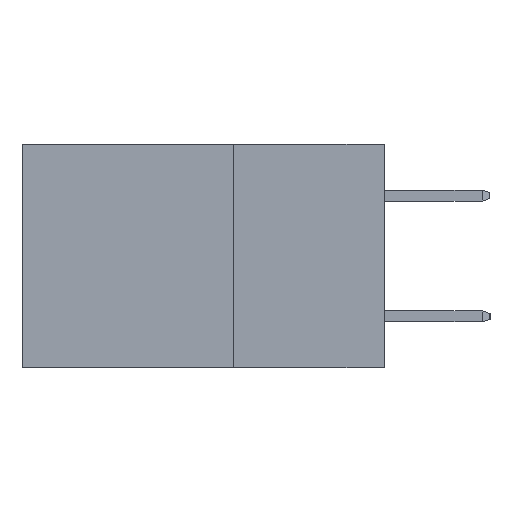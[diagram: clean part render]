
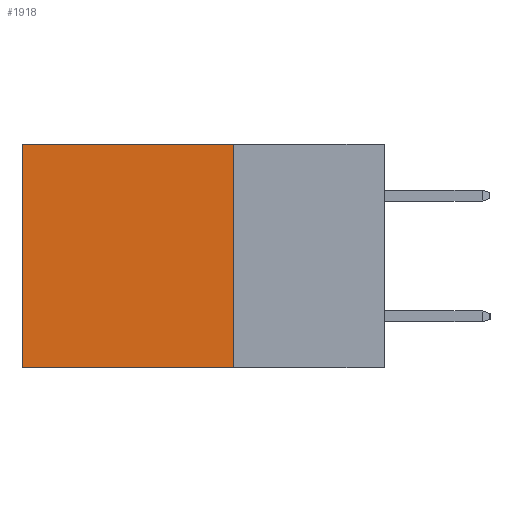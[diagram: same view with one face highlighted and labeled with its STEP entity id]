
A CAD part, left-side view. The second image highlights one B-rep face of the part: STEP entity #1918.
In plain terms, the highlighted planar face has unit normal (-1, 0, 0).
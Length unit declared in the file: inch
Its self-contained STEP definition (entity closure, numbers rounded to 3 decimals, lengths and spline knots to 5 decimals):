
#105 = FACE_OUTER_BOUND ( 'NONE', #2777, .T. ) ;
#188 = VECTOR ( 'NONE', #5989, 39.37008 ) ;
#465 = DIRECTION ( 'NONE',  ( 0., 0., -1. ) ) ;
#861 = VERTEX_POINT ( 'NONE', #7788 ) ;
#1149 = DIRECTION ( 'NONE',  ( 0., 0., -1. ) ) ;
#1711 = LINE ( 'NONE', #8958, #10531 ) ;
#1918 = ADVANCED_FACE ( 'NONE', ( #105 ), #6026, .F. ) ;
#2154 = EDGE_CURVE ( 'NONE', #5495, #8803, #7641, .T. ) ;
#2166 = ORIENTED_EDGE ( 'NONE', *, *, #3313, .T. ) ;
#2342 = CARTESIAN_POINT ( 'NONE',  ( 0.2615, 0.6, -0.37 ) ) ;
#2777 = EDGE_LOOP ( 'NONE', ( #4521, #6693, #10885, #2166 ) ) ;
#2877 = LINE ( 'NONE', #6540, #188 ) ;
#3112 = VECTOR ( 'NONE', #465, 39.37008 ) ;
#3313 = EDGE_CURVE ( 'NONE', #5495, #861, #5921, .T. ) ;
#4076 = EDGE_CURVE ( 'NONE', #8803, #6993, #1711, .T. ) ;
#4521 = ORIENTED_EDGE ( 'NONE', *, *, #7253, .T. ) ;
#4977 = CARTESIAN_POINT ( 'NONE',  ( 0.2615, 0.25, -0.37 ) ) ;
#5301 = DIRECTION ( 'NONE',  ( 1., 0., 0. ) ) ;
#5357 = CARTESIAN_POINT ( 'NONE',  ( 0.2615, 0.25, -0.37 ) ) ;
#5495 = VERTEX_POINT ( 'NONE', #6065 ) ;
#5921 = LINE ( 'NONE', #9659, #9849 ) ;
#5989 = DIRECTION ( 'NONE',  ( 0., 0., -1. ) ) ;
#6026 = PLANE ( 'NONE',  #6041 ) ;
#6041 = AXIS2_PLACEMENT_3D ( 'NONE', #11124, #5301, #1149 ) ;
#6065 = CARTESIAN_POINT ( 'NONE',  ( 0.2615, 0.25, 0. ) ) ;
#6540 = CARTESIAN_POINT ( 'NONE',  ( 0.2615, 0.6, -0.37 ) ) ;
#6693 = ORIENTED_EDGE ( 'NONE', *, *, #4076, .F. ) ;
#6993 = VERTEX_POINT ( 'NONE', #2342 ) ;
#7253 = EDGE_CURVE ( 'NONE', #861, #6993, #2877, .T. ) ;
#7641 = LINE ( 'NONE', #4977, #3112 ) ;
#7788 = CARTESIAN_POINT ( 'NONE',  ( 0.2615, 0.6, 0. ) ) ;
#8803 = VERTEX_POINT ( 'NONE', #5357 ) ;
#8958 = CARTESIAN_POINT ( 'NONE',  ( 0.2615, 0.25, -0.37 ) ) ;
#9454 = DIRECTION ( 'NONE',  ( 0., 1., 0. ) ) ;
#9659 = CARTESIAN_POINT ( 'NONE',  ( 0.2615, 0.25, 0. ) ) ;
#9764 = DIRECTION ( 'NONE',  ( 0., 1., 0. ) ) ;
#9849 = VECTOR ( 'NONE', #9764, 39.37008 ) ;
#10531 = VECTOR ( 'NONE', #9454, 39.37008 ) ;
#10885 = ORIENTED_EDGE ( 'NONE', *, *, #2154, .F. ) ;
#11124 = CARTESIAN_POINT ( 'NONE',  ( 0.2615, 0.25, -0.37 ) ) ;
